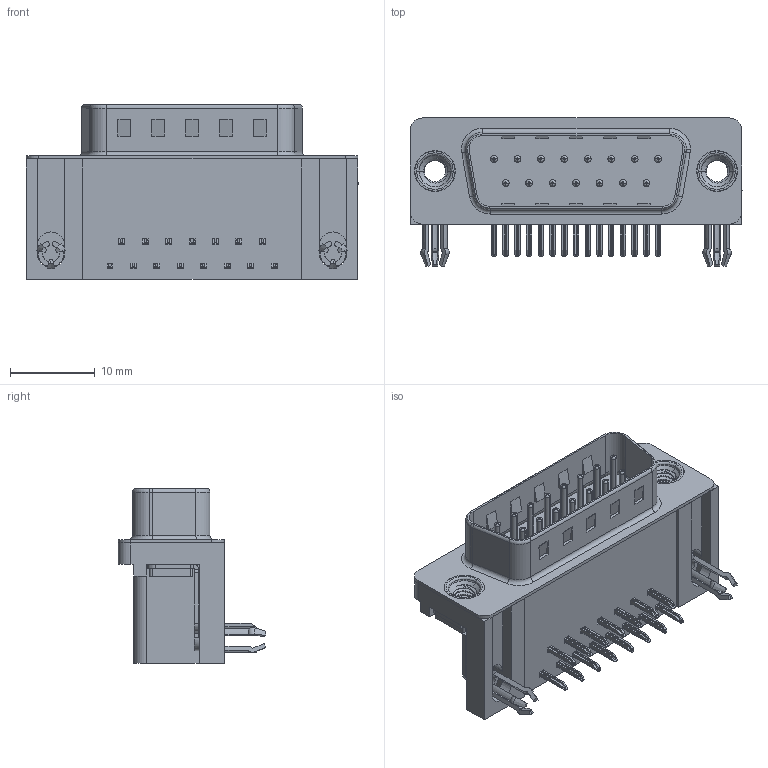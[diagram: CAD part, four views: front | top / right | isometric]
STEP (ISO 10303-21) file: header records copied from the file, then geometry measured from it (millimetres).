
FILE_DESCRIPTION (( 'STEP AP203' ), '1' );
FILE_NAME ('629-015-640-545.STEP', '2021-09-21T20:25:39', ( '' ), ( '' ), 'SwSTEP 2.0', 'SolidWorks 2020', '' );
FILE_SCHEMA (( 'CONFIG_CONTROL_DESIGN' ));
Length unit declared in the file: millimetre
Products named in the file (7): 629 Shell_15 Socket; 629 Contact Top; 629 Contact Bottom; 629 M3 Threaded Rivet; 629 3 Prong Board Lock; 629 Housing_15 Socket; 629-015-640-545
Assembly tree (21 placements, depth 2):
  629-015-640-545
    629 Housing_15 Socket
    629 Shell_15 Socket
    629 Contact Bottom  x7
    629 Contact Top  x8
    629 3 Prong Board Lock  x2
    629 M3 Threaded Rivet  x2
Bounding box: 39.22 x 17.48 x 20.6 mm (x, y, z)
Volume: 5083.8 mm3; surface area: 6136.5 mm2
Topology: 21 solids, 21 shells, 1579 faces, 3983 edges, 2483 vertices
Faces by surface type: plane 929, cylinder 455, torus 145, cone 44, bspline 6
Entity records: 20322 total; most frequent: CARTESIAN_POINT 4531, DIRECTION 3136, ORIENTED_EDGE 3008, EDGE_CURVE 1504, AXIS2_PLACEMENT_3D 1070, VECTOR 996, LINE 996, VERTEX_POINT 964
